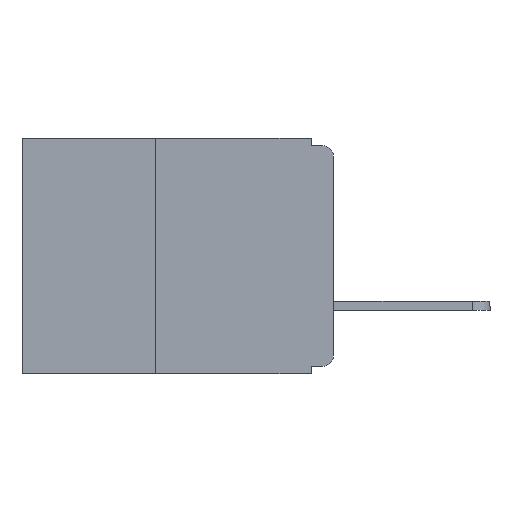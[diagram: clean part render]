
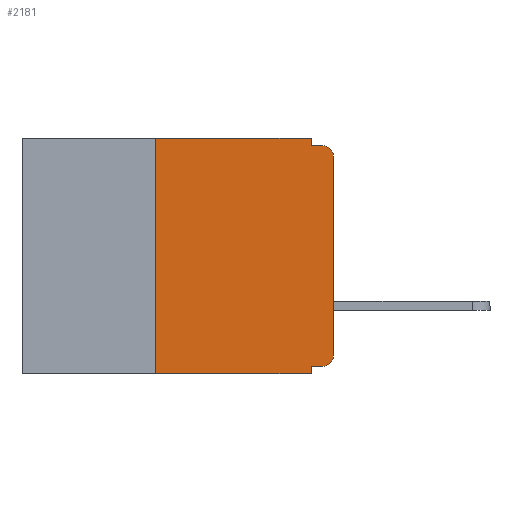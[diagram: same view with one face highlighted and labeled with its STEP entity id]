
A CAD part, left-side view. The second image highlights one B-rep face of the part: STEP entity #2181.
In plain terms, the highlighted planar face has unit normal (-1, 0, 0).
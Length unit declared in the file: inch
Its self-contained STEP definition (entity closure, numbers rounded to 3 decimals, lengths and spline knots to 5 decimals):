
#1834 = CIRCLE ( 'NONE', #27330, 0.015 ) ;
#2181 = ADVANCED_FACE ( 'NONE', ( #9880 ), #32327, .F. ) ;
#2316 = EDGE_CURVE ( 'NONE', #22228, #29306, #6583, .T. ) ;
#2839 = DIRECTION ( 'NONE',  ( 0., 0., -1. ) ) ;
#2907 = DIRECTION ( 'NONE',  ( 0., 0., 1. ) ) ;
#3100 = VERTEX_POINT ( 'NONE', #13025 ) ;
#3975 = VECTOR ( 'NONE', #8912, 39.37008 ) ;
#4295 = VECTOR ( 'NONE', #13632, 39.37008 ) ;
#4341 = CARTESIAN_POINT ( 'NONE',  ( 0., 0.031, 0. ) ) ;
#5094 = EDGE_CURVE ( 'NONE', #16281, #19062, #20459, .T. ) ;
#5397 = CARTESIAN_POINT ( 'NONE',  ( 0., 0.015, -0.32 ) ) ;
#5398 = EDGE_CURVE ( 'NONE', #22228, #15720, #5522, .T. ) ;
#5493 = VERTEX_POINT ( 'NONE', #11155 ) ;
#5522 = LINE ( 'NONE', #18586, #30909 ) ;
#5850 = EDGE_CURVE ( 'NONE', #19062, #17728, #31661, .T. ) ;
#6583 = CIRCLE ( 'NONE', #8862, 0.015 ) ;
#8034 = CARTESIAN_POINT ( 'NONE',  ( 0., 0.25, 0. ) ) ;
#8186 = VECTOR ( 'NONE', #2907, 39.37008 ) ;
#8862 = AXIS2_PLACEMENT_3D ( 'NONE', #28724, #28655, #28554 ) ;
#8912 = DIRECTION ( 'NONE',  ( 0., 0., -1. ) ) ;
#9880 = FACE_OUTER_BOUND ( 'NONE', #29867, .T. ) ;
#10045 = DIRECTION ( 'NONE',  ( 0., 0., 1. ) ) ;
#10402 = DIRECTION ( 'NONE',  ( 0., -1., 0. ) ) ;
#10796 = CARTESIAN_POINT ( 'NONE',  ( 0., 0.25, -0.33 ) ) ;
#11155 = CARTESIAN_POINT ( 'NONE',  ( 0., 0., -0.025 ) ) ;
#11255 = LINE ( 'NONE', #28656, #4295 ) ;
#11269 = CARTESIAN_POINT ( 'NONE',  ( 0., 0., -0.305 ) ) ;
#11851 = DIRECTION ( 'NONE',  ( -1., 0., 0. ) ) ;
#11924 = ORIENTED_EDGE ( 'NONE', *, *, #17886, .T. ) ;
#13025 = CARTESIAN_POINT ( 'NONE',  ( 0., 0.031, -0.33 ) ) ;
#13632 = DIRECTION ( 'NONE',  ( 0., -1., 0. ) ) ;
#13718 = VECTOR ( 'NONE', #2839, 39.37008 ) ;
#14302 = ORIENTED_EDGE ( 'NONE', *, *, #5094, .F. ) ;
#15015 = ORIENTED_EDGE ( 'NONE', *, *, #28038, .T. ) ;
#15207 = ORIENTED_EDGE ( 'NONE', *, *, #15299, .F. ) ;
#15299 = EDGE_CURVE ( 'NONE', #15720, #3100, #18601, .T. ) ;
#15646 = CARTESIAN_POINT ( 'NONE',  ( 0., 0.031, -0.01 ) ) ;
#15720 = VERTEX_POINT ( 'NONE', #22746 ) ;
#16164 = VECTOR ( 'NONE', #10045, 39.37008 ) ;
#16281 = VERTEX_POINT ( 'NONE', #24782 ) ;
#17728 = VERTEX_POINT ( 'NONE', #23707 ) ;
#17886 = EDGE_CURVE ( 'NONE', #5493, #17728, #1834, .T. ) ;
#18586 = CARTESIAN_POINT ( 'NONE',  ( 0., 0., -0.32 ) ) ;
#18601 = LINE ( 'NONE', #24139, #3975 ) ;
#18807 = ORIENTED_EDGE ( 'NONE', *, *, #29018, .F. ) ;
#19062 = VERTEX_POINT ( 'NONE', #15646 ) ;
#19339 = ORIENTED_EDGE ( 'NONE', *, *, #5850, .F. ) ;
#19460 = DIRECTION ( 'NONE',  ( 0., 1., 0. ) ) ;
#20199 = EDGE_CURVE ( 'NONE', #29306, #5493, #21778, .T. ) ;
#20250 = VERTEX_POINT ( 'NONE', #10796 ) ;
#20459 = LINE ( 'NONE', #4341, #13718 ) ;
#21778 = LINE ( 'NONE', #28351, #8186 ) ;
#22041 = LINE ( 'NONE', #25227, #16164 ) ;
#22113 = LINE ( 'NONE', #25575, #27942 ) ;
#22228 = VERTEX_POINT ( 'NONE', #5397 ) ;
#22746 = CARTESIAN_POINT ( 'NONE',  ( 0., 0.031, -0.32 ) ) ;
#23705 = ORIENTED_EDGE ( 'NONE', *, *, #5398, .F. ) ;
#23707 = CARTESIAN_POINT ( 'NONE',  ( 0., 0.015, -0.01 ) ) ;
#24139 = CARTESIAN_POINT ( 'NONE',  ( 0., 0.031, -0.33 ) ) ;
#24319 = VECTOR ( 'NONE', #25404, 39.37008 ) ;
#24738 = ORIENTED_EDGE ( 'NONE', *, *, #26733, .F. ) ;
#24782 = CARTESIAN_POINT ( 'NONE',  ( 0., 0.031, 0. ) ) ;
#25227 = CARTESIAN_POINT ( 'NONE',  ( 0., 0.25, -0.33 ) ) ;
#25404 = DIRECTION ( 'NONE',  ( 0., -1., 0. ) ) ;
#25509 = CARTESIAN_POINT ( 'NONE',  ( 0., 0., -0.01 ) ) ;
#25575 = CARTESIAN_POINT ( 'NONE',  ( 0., 0.437, 0. ) ) ;
#26513 = AXIS2_PLACEMENT_3D ( 'NONE', #32184, #31928, #31764 ) ;
#26628 = ORIENTED_EDGE ( 'NONE', *, *, #2316, .T. ) ;
#26733 = EDGE_CURVE ( 'NONE', #31372, #16281, #22113, .T. ) ;
#26991 = CARTESIAN_POINT ( 'NONE',  ( 0., 0.015, -0.025 ) ) ;
#27330 = AXIS2_PLACEMENT_3D ( 'NONE', #26991, #11851, #29448 ) ;
#27942 = VECTOR ( 'NONE', #10402, 39.37008 ) ;
#28038 = EDGE_CURVE ( 'NONE', #20250, #3100, #11255, .T. ) ;
#28351 = CARTESIAN_POINT ( 'NONE',  ( 0., 0., 0. ) ) ;
#28554 = DIRECTION ( 'NONE',  ( 0., 0., -1. ) ) ;
#28655 = DIRECTION ( 'NONE',  ( -1., 0., 0. ) ) ;
#28656 = CARTESIAN_POINT ( 'NONE',  ( 0., 0.437, -0.33 ) ) ;
#28724 = CARTESIAN_POINT ( 'NONE',  ( 0., 0.015, -0.305 ) ) ;
#29018 = EDGE_CURVE ( 'NONE', #20250, #31372, #22041, .T. ) ;
#29306 = VERTEX_POINT ( 'NONE', #11269 ) ;
#29448 = DIRECTION ( 'NONE',  ( 0., 0., -1. ) ) ;
#29867 = EDGE_LOOP ( 'NONE', ( #32417, #11924, #19339, #14302, #24738, #18807, #15015, #15207, #23705, #26628 ) ) ;
#30909 = VECTOR ( 'NONE', #19460, 39.37008 ) ;
#31372 = VERTEX_POINT ( 'NONE', #8034 ) ;
#31661 = LINE ( 'NONE', #25509, #24319 ) ;
#31764 = DIRECTION ( 'NONE',  ( 0., 0., -1. ) ) ;
#31928 = DIRECTION ( 'NONE',  ( 1., 0., 0. ) ) ;
#32184 = CARTESIAN_POINT ( 'NONE',  ( 0., 0.437, 0. ) ) ;
#32327 = PLANE ( 'NONE',  #26513 ) ;
#32417 = ORIENTED_EDGE ( 'NONE', *, *, #20199, .T. ) ;
